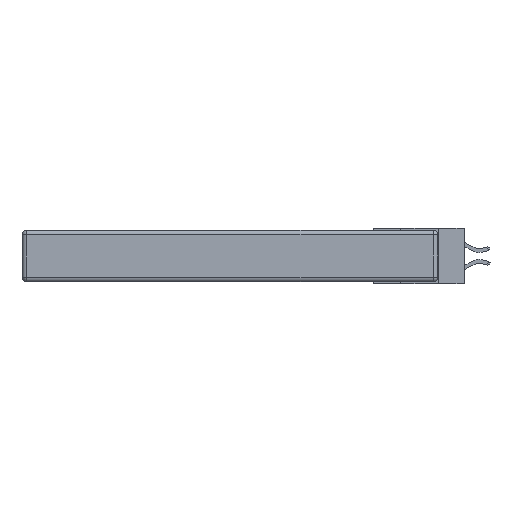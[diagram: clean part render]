
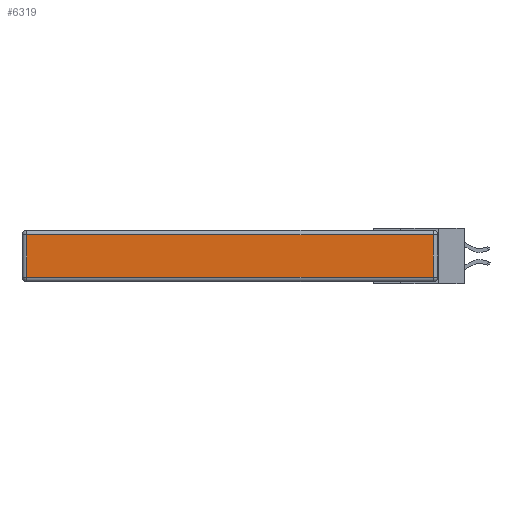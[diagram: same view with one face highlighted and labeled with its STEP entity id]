
A CAD part, left-side view. The second image highlights one B-rep face of the part: STEP entity #6319.
In plain terms, the highlighted planar face has unit normal (-1, 0, 0).
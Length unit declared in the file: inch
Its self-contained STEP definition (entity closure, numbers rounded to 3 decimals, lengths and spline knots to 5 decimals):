
#750 = CARTESIAN_POINT ( 'NONE',  ( 0., 2.75, -0.03 ) ) ;
#1109 = CARTESIAN_POINT ( 'NONE',  ( 0., 0., -0.313 ) ) ;
#1758 = CARTESIAN_POINT ( 'NONE',  ( 0., 2.72, -0.03 ) ) ;
#2321 = ORIENTED_EDGE ( 'NONE', *, *, #24764, .T. ) ;
#3203 = DIRECTION ( 'NONE',  ( 0., -1., 0. ) ) ;
#3716 = VERTEX_POINT ( 'NONE', #4699 ) ;
#3728 = CARTESIAN_POINT ( 'NONE',  ( 0., 0., -0.343 ) ) ;
#4699 = CARTESIAN_POINT ( 'NONE',  ( 0., 0.03, -0.03 ) ) ;
#6319 = ADVANCED_FACE ( 'NONE', ( #10907 ), #19534, .T. ) ;
#8244 = EDGE_LOOP ( 'NONE', ( #23250, #2321, #16417, #13973 ) ) ;
#9696 = VECTOR ( 'NONE', #12730, 39.37008 ) ;
#10505 = LINE ( 'NONE', #750, #10803 ) ;
#10803 = VECTOR ( 'NONE', #17113, 39.37008 ) ;
#10907 = FACE_OUTER_BOUND ( 'NONE', #8244, .T. ) ;
#11523 = CARTESIAN_POINT ( 'NONE',  ( 0., 2.72, -0.313 ) ) ;
#11711 = VECTOR ( 'NONE', #18833, 39.37008 ) ;
#12730 = DIRECTION ( 'NONE',  ( 0., 0., -1. ) ) ;
#13797 = AXIS2_PLACEMENT_3D ( 'NONE', #3728, #21478, #19691 ) ;
#13804 = LINE ( 'NONE', #20621, #9696 ) ;
#13973 = ORIENTED_EDGE ( 'NONE', *, *, #19377, .T. ) ;
#14113 = EDGE_CURVE ( 'NONE', #25601, #14813, #22848, .T. ) ;
#14519 = LINE ( 'NONE', #24876, #11711 ) ;
#14813 = VERTEX_POINT ( 'NONE', #18367 ) ;
#16417 = ORIENTED_EDGE ( 'NONE', *, *, #24305, .T. ) ;
#17113 = DIRECTION ( 'NONE',  ( 0., 1., 0. ) ) ;
#18367 = CARTESIAN_POINT ( 'NONE',  ( 0., 0.03, -0.313 ) ) ;
#18833 = DIRECTION ( 'NONE',  ( 0., 0., 1. ) ) ;
#19377 = EDGE_CURVE ( 'NONE', #21384, #25601, #13804, .T. ) ;
#19534 = PLANE ( 'NONE',  #13797 ) ;
#19691 = DIRECTION ( 'NONE',  ( 0., 0., 1. ) ) ;
#20621 = CARTESIAN_POINT ( 'NONE',  ( 0., 2.72, -0.343 ) ) ;
#21384 = VERTEX_POINT ( 'NONE', #1758 ) ;
#21478 = DIRECTION ( 'NONE',  ( -1., 0., 0. ) ) ;
#21573 = VECTOR ( 'NONE', #3203, 39.37008 ) ;
#22848 = LINE ( 'NONE', #1109, #21573 ) ;
#23250 = ORIENTED_EDGE ( 'NONE', *, *, #14113, .T. ) ;
#24305 = EDGE_CURVE ( 'NONE', #3716, #21384, #10505, .T. ) ;
#24764 = EDGE_CURVE ( 'NONE', #14813, #3716, #14519, .T. ) ;
#24876 = CARTESIAN_POINT ( 'NONE',  ( 0., 0.03, -0.343 ) ) ;
#25601 = VERTEX_POINT ( 'NONE', #11523 ) ;
